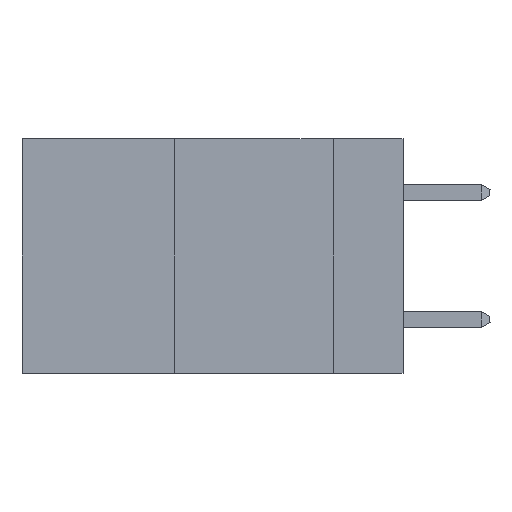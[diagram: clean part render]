
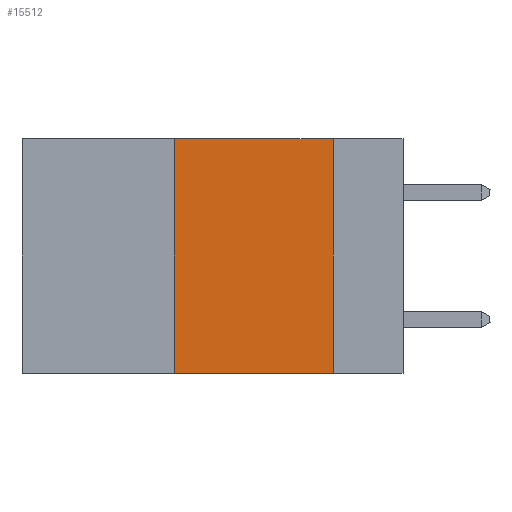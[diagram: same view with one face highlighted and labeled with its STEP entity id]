
A CAD part, left-side view. The second image highlights one B-rep face of the part: STEP entity #15512.
In plain terms, the highlighted planar face has unit normal (-1, 0, 0).
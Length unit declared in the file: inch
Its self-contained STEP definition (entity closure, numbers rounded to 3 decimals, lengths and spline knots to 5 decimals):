
#1226 = CARTESIAN_POINT ( 'NONE',  ( 0., 0.6, 0. ) ) ;
#1389 = VECTOR ( 'NONE', #4756, 39.37008 ) ;
#1411 = DIRECTION ( 'NONE',  ( 0., 0., 1. ) ) ;
#3611 = AXIS2_PLACEMENT_3D ( 'NONE', #35401, #14732, #38902 ) ;
#4756 = DIRECTION ( 'NONE',  ( 0., -1., 0. ) ) ;
#5173 = FACE_OUTER_BOUND ( 'NONE', #15745, .T. ) ;
#6057 = CARTESIAN_POINT ( 'NONE',  ( 0., 0.6, -0.37 ) ) ;
#6916 = VERTEX_POINT ( 'NONE', #34376 ) ;
#7749 = PLANE ( 'NONE',  #3611 ) ;
#9168 = DIRECTION ( 'NONE',  ( 0., 0., -1. ) ) ;
#9229 = ORIENTED_EDGE ( 'NONE', *, *, #19161, .T. ) ;
#10227 = VERTEX_POINT ( 'NONE', #28608 ) ;
#10692 = CARTESIAN_POINT ( 'NONE',  ( 0., 0.11, 0. ) ) ;
#13200 = VERTEX_POINT ( 'NONE', #36446 ) ;
#13861 = LINE ( 'NONE', #42885, #21926 ) ;
#14531 = EDGE_CURVE ( 'NONE', #33335, #10227, #26882, .T. ) ;
#14732 = DIRECTION ( 'NONE',  ( 1., 0., 0. ) ) ;
#15512 = ADVANCED_FACE ( 'NONE', ( #5173 ), #7749, .F. ) ;
#15560 = VECTOR ( 'NONE', #9168, 39.37008 ) ;
#15745 = EDGE_LOOP ( 'NONE', ( #20618, #43533, #17517, #9229 ) ) ;
#16490 = DIRECTION ( 'NONE',  ( 0., -1., 0. ) ) ;
#17517 = ORIENTED_EDGE ( 'NONE', *, *, #33008, .F. ) ;
#19161 = EDGE_CURVE ( 'NONE', #6916, #10227, #41071, .T. ) ;
#20618 = ORIENTED_EDGE ( 'NONE', *, *, #14531, .F. ) ;
#21926 = VECTOR ( 'NONE', #1411, 39.37008 ) ;
#23753 = VECTOR ( 'NONE', #16490, 39.37008 ) ;
#26882 = LINE ( 'NONE', #36825, #15560 ) ;
#28608 = CARTESIAN_POINT ( 'NONE',  ( 0., 0.11, -0.37 ) ) ;
#29006 = LINE ( 'NONE', #1226, #1389 ) ;
#29771 = EDGE_CURVE ( 'NONE', #13200, #33335, #29006, .T. ) ;
#33008 = EDGE_CURVE ( 'NONE', #6916, #13200, #13861, .T. ) ;
#33335 = VERTEX_POINT ( 'NONE', #10692 ) ;
#34376 = CARTESIAN_POINT ( 'NONE',  ( 0., 0.36, -0.37 ) ) ;
#35401 = CARTESIAN_POINT ( 'NONE',  ( 0., 0.6, 0. ) ) ;
#36446 = CARTESIAN_POINT ( 'NONE',  ( 0., 0.36, 0. ) ) ;
#36825 = CARTESIAN_POINT ( 'NONE',  ( 0., 0.11, 0. ) ) ;
#38902 = DIRECTION ( 'NONE',  ( 0., 0., -1. ) ) ;
#41071 = LINE ( 'NONE', #6057, #23753 ) ;
#42885 = CARTESIAN_POINT ( 'NONE',  ( 0., 0.36, 0. ) ) ;
#43533 = ORIENTED_EDGE ( 'NONE', *, *, #29771, .F. ) ;
